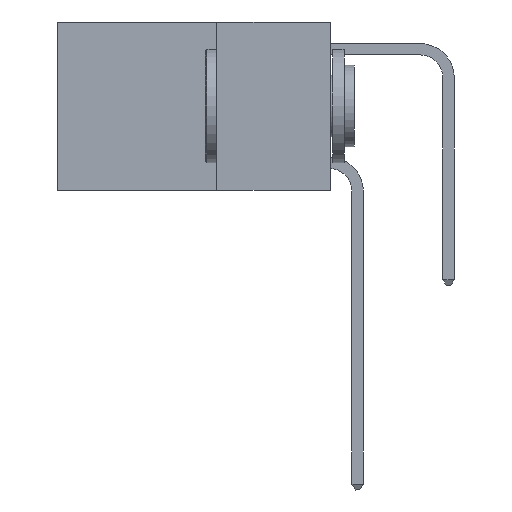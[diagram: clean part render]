
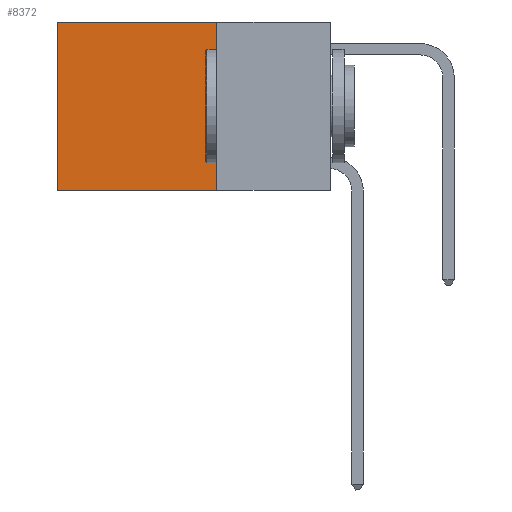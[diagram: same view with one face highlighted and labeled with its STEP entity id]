
A CAD part, left-side view. The second image highlights one B-rep face of the part: STEP entity #8372.
In plain terms, the highlighted planar face has unit normal (-1, 0, 0).
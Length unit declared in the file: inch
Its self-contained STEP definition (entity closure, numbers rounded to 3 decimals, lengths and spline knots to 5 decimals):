
#753 = LINE ( 'NONE', #8535, #5512 ) ;
#759 = CARTESIAN_POINT ( 'NONE',  ( 0.2625, 0.25, 0. ) ) ;
#894 = VERTEX_POINT ( 'NONE', #759 ) ;
#1448 = AXIS2_PLACEMENT_3D ( 'NONE', #9975, #3936, #2920 ) ;
#1673 = EDGE_CURVE ( 'NONE', #894, #7929, #10182, .T. ) ;
#1684 = LINE ( 'NONE', #10739, #8445 ) ;
#2307 = DIRECTION ( 'NONE',  ( 0., 0., -1. ) ) ;
#2891 = ORIENTED_EDGE ( 'NONE', *, *, #1673, .T. ) ;
#2920 = DIRECTION ( 'NONE',  ( 0., 0., -1. ) ) ;
#3104 = FACE_OUTER_BOUND ( 'NONE', #10533, .T. ) ;
#3400 = ORIENTED_EDGE ( 'NONE', *, *, #12334, .F. ) ;
#3447 = VECTOR ( 'NONE', #2307, 39.37008 ) ;
#3936 = DIRECTION ( 'NONE',  ( 1., 0., 0. ) ) ;
#4603 = DIRECTION ( 'NONE',  ( 0., 1., 0. ) ) ;
#5461 = VECTOR ( 'NONE', #6107, 39.37008 ) ;
#5512 = VECTOR ( 'NONE', #4603, 39.37008 ) ;
#5601 = ORIENTED_EDGE ( 'NONE', *, *, #6250, .F. ) ;
#6107 = DIRECTION ( 'NONE',  ( 0., 1., 0. ) ) ;
#6186 = EDGE_CURVE ( 'NONE', #7929, #8755, #7348, .T. ) ;
#6250 = EDGE_CURVE ( 'NONE', #7636, #8755, #753, .T. ) ;
#6448 = CARTESIAN_POINT ( 'NONE',  ( 0.2625, 0.6, 0. ) ) ;
#7138 = PLANE ( 'NONE',  #1448 ) ;
#7348 = LINE ( 'NONE', #6448, #3447 ) ;
#7584 = DIRECTION ( 'NONE',  ( 0., 0., -1. ) ) ;
#7636 = VERTEX_POINT ( 'NONE', #9445 ) ;
#7929 = VERTEX_POINT ( 'NONE', #11397 ) ;
#8155 = CARTESIAN_POINT ( 'NONE',  ( 0.2625, 0.25, 0. ) ) ;
#8372 = ADVANCED_FACE ( 'NONE', ( #3104 ), #7138, .F. ) ;
#8445 = VECTOR ( 'NONE', #7584, 39.37008 ) ;
#8535 = CARTESIAN_POINT ( 'NONE',  ( 0.2625, 0.25, -0.37 ) ) ;
#8755 = VERTEX_POINT ( 'NONE', #10199 ) ;
#9445 = CARTESIAN_POINT ( 'NONE',  ( 0.2625, 0.25, -0.37 ) ) ;
#9975 = CARTESIAN_POINT ( 'NONE',  ( 0.2625, 0.25, 0. ) ) ;
#10182 = LINE ( 'NONE', #8155, #5461 ) ;
#10199 = CARTESIAN_POINT ( 'NONE',  ( 0.2625, 0.6, -0.37 ) ) ;
#10533 = EDGE_LOOP ( 'NONE', ( #11593, #5601, #3400, #2891 ) ) ;
#10739 = CARTESIAN_POINT ( 'NONE',  ( 0.2625, 0.25, 0. ) ) ;
#11397 = CARTESIAN_POINT ( 'NONE',  ( 0.2625, 0.6, 0. ) ) ;
#11593 = ORIENTED_EDGE ( 'NONE', *, *, #6186, .T. ) ;
#12334 = EDGE_CURVE ( 'NONE', #894, #7636, #1684, .T. ) ;
